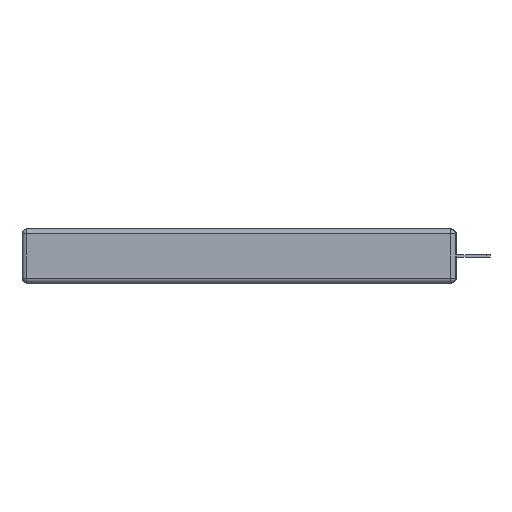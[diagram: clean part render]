
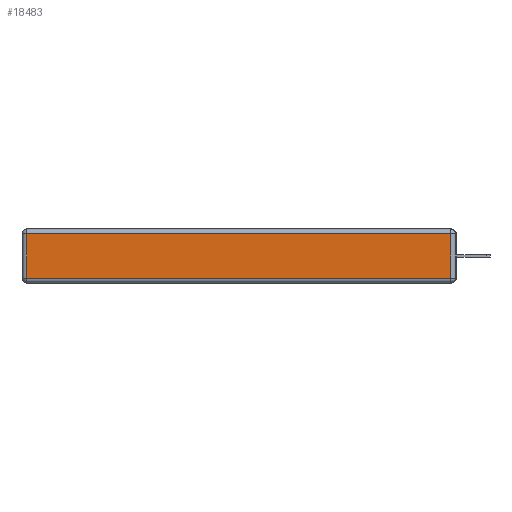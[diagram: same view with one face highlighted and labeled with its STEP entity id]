
A CAD part, left-side view. The second image highlights one B-rep face of the part: STEP entity #18483.
In plain terms, the highlighted planar face has unit normal (-1, 0, 0).
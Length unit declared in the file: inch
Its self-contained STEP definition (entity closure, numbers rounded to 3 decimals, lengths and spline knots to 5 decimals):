
#137 = AXIS2_PLACEMENT_3D ( 'NONE', #12960, #28992, #15229 ) ;
#730 = DIRECTION ( 'NONE',  ( 0., 0., -1. ) ) ;
#953 = CARTESIAN_POINT ( 'NONE',  ( 0., 0., -0.313 ) ) ;
#1189 = VECTOR ( 'NONE', #17569, 39.37008 ) ;
#3902 = CARTESIAN_POINT ( 'NONE',  ( 0., 0.03, -0.343 ) ) ;
#5022 = VECTOR ( 'NONE', #28177, 39.37008 ) ;
#6006 = VERTEX_POINT ( 'NONE', #23608 ) ;
#6076 = PLANE ( 'NONE',  #137 ) ;
#7194 = EDGE_LOOP ( 'NONE', ( #15350, #9355, #17383, #20546 ) ) ;
#8042 = DIRECTION ( 'NONE',  ( 0., -1., 0. ) ) ;
#8481 = CARTESIAN_POINT ( 'NONE',  ( 0., 2.72, -0.313 ) ) ;
#9355 = ORIENTED_EDGE ( 'NONE', *, *, #25657, .T. ) ;
#9761 = EDGE_CURVE ( 'NONE', #20470, #6006, #10809, .T. ) ;
#10407 = LINE ( 'NONE', #14435, #5022 ) ;
#10809 = LINE ( 'NONE', #953, #29064 ) ;
#12336 = VERTEX_POINT ( 'NONE', #13074 ) ;
#12950 = VECTOR ( 'NONE', #730, 39.37008 ) ;
#12960 = CARTESIAN_POINT ( 'NONE',  ( 0., 0., -0.343 ) ) ;
#13074 = CARTESIAN_POINT ( 'NONE',  ( 0., 0.03, -0.03 ) ) ;
#14435 = CARTESIAN_POINT ( 'NONE',  ( 0., 2.75, -0.03 ) ) ;
#15229 = DIRECTION ( 'NONE',  ( 0., 0., 1. ) ) ;
#15350 = ORIENTED_EDGE ( 'NONE', *, *, #9761, .T. ) ;
#17383 = ORIENTED_EDGE ( 'NONE', *, *, #23772, .T. ) ;
#17569 = DIRECTION ( 'NONE',  ( 0., 0., 1. ) ) ;
#18483 = ADVANCED_FACE ( 'NONE', ( #23862 ), #6076, .T. ) ;
#18793 = LINE ( 'NONE', #3902, #1189 ) ;
#18983 = LINE ( 'NONE', #21347, #12950 ) ;
#20470 = VERTEX_POINT ( 'NONE', #8481 ) ;
#20546 = ORIENTED_EDGE ( 'NONE', *, *, #21869, .T. ) ;
#20871 = VERTEX_POINT ( 'NONE', #23684 ) ;
#21347 = CARTESIAN_POINT ( 'NONE',  ( 0., 2.72, -0.343 ) ) ;
#21869 = EDGE_CURVE ( 'NONE', #20871, #20470, #18983, .T. ) ;
#23608 = CARTESIAN_POINT ( 'NONE',  ( 0., 0.03, -0.313 ) ) ;
#23684 = CARTESIAN_POINT ( 'NONE',  ( 0., 2.72, -0.03 ) ) ;
#23772 = EDGE_CURVE ( 'NONE', #12336, #20871, #10407, .T. ) ;
#23862 = FACE_OUTER_BOUND ( 'NONE', #7194, .T. ) ;
#25657 = EDGE_CURVE ( 'NONE', #6006, #12336, #18793, .T. ) ;
#28177 = DIRECTION ( 'NONE',  ( 0., 1., 0. ) ) ;
#28992 = DIRECTION ( 'NONE',  ( -1., 0., 0. ) ) ;
#29064 = VECTOR ( 'NONE', #8042, 39.37008 ) ;
